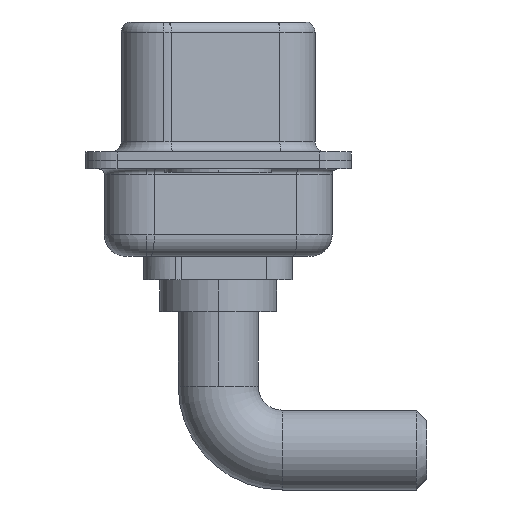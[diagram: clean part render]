
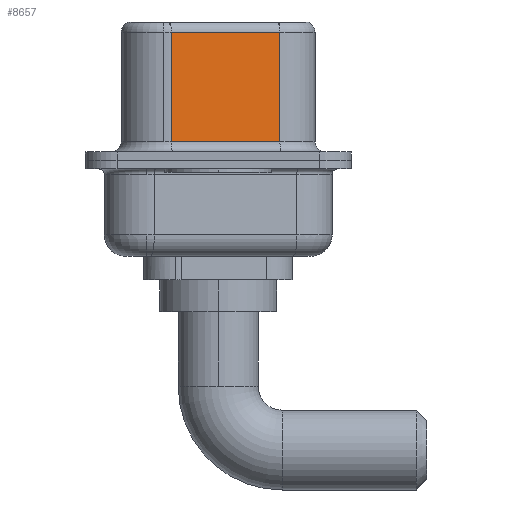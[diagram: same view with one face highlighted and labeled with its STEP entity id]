
A CAD part, left-side view. The second image highlights one B-rep face of the part: STEP entity #8657.
In plain terms, the highlighted planar face has unit normal (-0.985, -0.174, 0).
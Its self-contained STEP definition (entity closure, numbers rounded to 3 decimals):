
#712 = DIRECTION ( 'NONE',  ( 0.985, 0.174, 0. ) ) ;
#847 = AXIS2_PLACEMENT_3D ( 'NONE', #11821, #712, #12769 ) ;
#1257 = CARTESIAN_POINT ( 'NONE',  ( 4.58, -2.897, 6.52 ) ) ;
#2382 = ORIENTED_EDGE ( 'NONE', *, *, #12751, .F. ) ;
#2706 = VERTEX_POINT ( 'NONE', #7574 ) ;
#3176 = CARTESIAN_POINT ( 'NONE',  ( 3.68, 2.203, 0.9 ) ) ;
#3854 = VECTOR ( 'NONE', #13597, 1000. ) ;
#4257 = CARTESIAN_POINT ( 'NONE',  ( 3.68, 2.203, 6.52 ) ) ;
#4480 = CARTESIAN_POINT ( 'NONE',  ( 4.58, -2.897, 6.02 ) ) ;
#4488 = VECTOR ( 'NONE', #9307, 1000. ) ;
#4712 = ORIENTED_EDGE ( 'NONE', *, *, #7255, .T. ) ;
#4739 = CARTESIAN_POINT ( 'NONE',  ( 4.58, -2.897, 0.9 ) ) ;
#4929 = CARTESIAN_POINT ( 'NONE',  ( 4.58, -2.897, 0.9 ) ) ;
#5793 = LINE ( 'NONE', #5861, #3854 ) ;
#5861 = CARTESIAN_POINT ( 'NONE',  ( 4.58, -2.897, 6.02 ) ) ;
#6998 = LINE ( 'NONE', #4739, #4488 ) ;
#7146 = VECTOR ( 'NONE', #8994, 1000. ) ;
#7255 = EDGE_CURVE ( 'NONE', #10652, #8281, #6998, .T. ) ;
#7574 = CARTESIAN_POINT ( 'NONE',  ( 3.68, 2.203, 6.02 ) ) ;
#8281 = VERTEX_POINT ( 'NONE', #4929 ) ;
#8439 = PLANE ( 'NONE',  #847 ) ;
#8657 = ADVANCED_FACE ( 'NONE', ( #10614 ), #8439, .F. ) ;
#8994 = DIRECTION ( 'NONE',  ( 0., 0., -1. ) ) ;
#9163 = EDGE_CURVE ( 'NONE', #10719, #2706, #5793, .T. ) ;
#9214 = LINE ( 'NONE', #1257, #7146 ) ;
#9307 = DIRECTION ( 'NONE',  ( 0.174, -0.985, 0. ) ) ;
#9475 = EDGE_CURVE ( 'NONE', #2706, #10652, #10849, .T. ) ;
#9728 = EDGE_LOOP ( 'NONE', ( #2382, #10361, #12506, #4712 ) ) ;
#10361 = ORIENTED_EDGE ( 'NONE', *, *, #9163, .T. ) ;
#10614 = FACE_OUTER_BOUND ( 'NONE', #9728, .T. ) ;
#10652 = VERTEX_POINT ( 'NONE', #3176 ) ;
#10719 = VERTEX_POINT ( 'NONE', #4480 ) ;
#10849 = LINE ( 'NONE', #4257, #11721 ) ;
#11721 = VECTOR ( 'NONE', #12866, 1000. ) ;
#11821 = CARTESIAN_POINT ( 'NONE',  ( 4.58, -2.897, 6.52 ) ) ;
#12506 = ORIENTED_EDGE ( 'NONE', *, *, #9475, .T. ) ;
#12751 = EDGE_CURVE ( 'NONE', #10719, #8281, #9214, .T. ) ;
#12769 = DIRECTION ( 'NONE',  ( -0.174, 0.985, 0. ) ) ;
#12866 = DIRECTION ( 'NONE',  ( 0., 0., -1. ) ) ;
#13597 = DIRECTION ( 'NONE',  ( -0.174, 0.985, 0. ) ) ;
